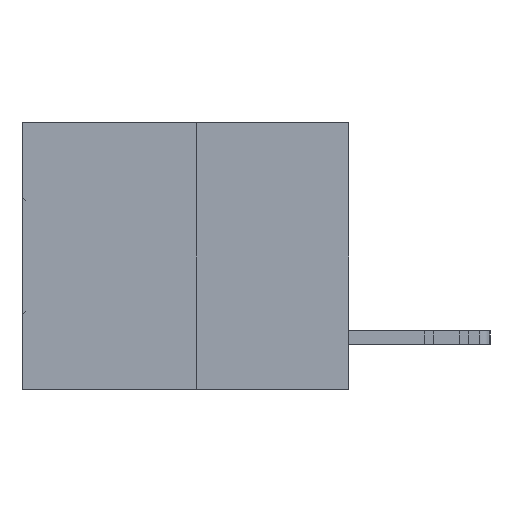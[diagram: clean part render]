
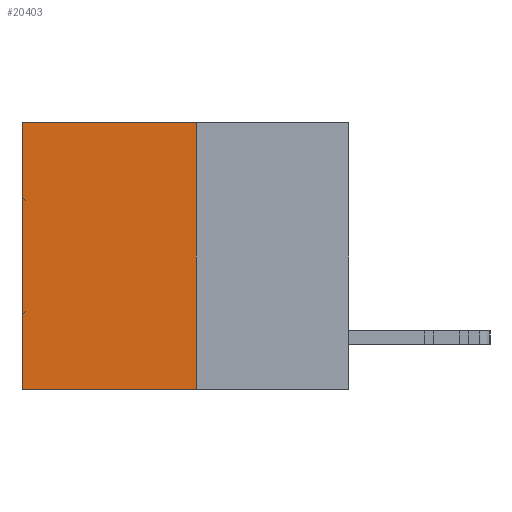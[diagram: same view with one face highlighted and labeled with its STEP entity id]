
A CAD part, left-side view. The second image highlights one B-rep face of the part: STEP entity #20403.
In plain terms, the highlighted planar face has unit normal (-1, 0, 0).
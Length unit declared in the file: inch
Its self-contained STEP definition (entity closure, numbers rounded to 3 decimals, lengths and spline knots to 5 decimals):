
#123 = LINE ( 'NONE', #18895, #16174 ) ;
#793 = CARTESIAN_POINT ( 'NONE',  ( 0.3165, 0.28, -0.49 ) ) ;
#831 = LINE ( 'NONE', #4594, #22726 ) ;
#1017 = LINE ( 'NONE', #18069, #3872 ) ;
#1722 = CARTESIAN_POINT ( 'NONE',  ( 0.3165, 0.6, -0.49 ) ) ;
#2252 = DIRECTION ( 'NONE',  ( 0., 0., -1. ) ) ;
#3872 = VECTOR ( 'NONE', #2252, 39.37008 ) ;
#4594 = CARTESIAN_POINT ( 'NONE',  ( 0.3165, 0.28, 0. ) ) ;
#9068 = VERTEX_POINT ( 'NONE', #22240 ) ;
#10817 = CARTESIAN_POINT ( 'NONE',  ( 0.3165, 0.28, -0.49 ) ) ;
#12361 = CARTESIAN_POINT ( 'NONE',  ( 0.3165, 0.28, 0. ) ) ;
#13529 = EDGE_LOOP ( 'NONE', ( #17844, #29411, #20712, #14182 ) ) ;
#13698 = VERTEX_POINT ( 'NONE', #14659 ) ;
#13804 = PLANE ( 'NONE',  #16335 ) ;
#14182 = ORIENTED_EDGE ( 'NONE', *, *, #19630, .T. ) ;
#14659 = CARTESIAN_POINT ( 'NONE',  ( 0.3165, 0.6, 0. ) ) ;
#15129 = EDGE_CURVE ( 'NONE', #34155, #26546, #1017, .T. ) ;
#15660 = VECTOR ( 'NONE', #21208, 39.37008 ) ;
#16174 = VECTOR ( 'NONE', #24242, 39.37008 ) ;
#16335 = AXIS2_PLACEMENT_3D ( 'NONE', #793, #19218, #21887 ) ;
#16602 = EDGE_CURVE ( 'NONE', #26546, #9068, #123, .T. ) ;
#17844 = ORIENTED_EDGE ( 'NONE', *, *, #31906, .T. ) ;
#18069 = CARTESIAN_POINT ( 'NONE',  ( 0.3165, 0.28, -0.49 ) ) ;
#18895 = CARTESIAN_POINT ( 'NONE',  ( 0.3165, 0.28, -0.49 ) ) ;
#19218 = DIRECTION ( 'NONE',  ( 1., 0., 0. ) ) ;
#19630 = EDGE_CURVE ( 'NONE', #34155, #13698, #831, .T. ) ;
#20403 = ADVANCED_FACE ( 'NONE', ( #25981 ), #13804, .F. ) ;
#20712 = ORIENTED_EDGE ( 'NONE', *, *, #15129, .F. ) ;
#21208 = DIRECTION ( 'NONE',  ( 0., 0., -1. ) ) ;
#21887 = DIRECTION ( 'NONE',  ( 0., 0., -1. ) ) ;
#22240 = CARTESIAN_POINT ( 'NONE',  ( 0.3165, 0.6, -0.49 ) ) ;
#22726 = VECTOR ( 'NONE', #28234, 39.37008 ) ;
#22733 = LINE ( 'NONE', #1722, #15660 ) ;
#24242 = DIRECTION ( 'NONE',  ( 0., 1., 0. ) ) ;
#25981 = FACE_OUTER_BOUND ( 'NONE', #13529, .T. ) ;
#26546 = VERTEX_POINT ( 'NONE', #10817 ) ;
#28234 = DIRECTION ( 'NONE',  ( 0., 1., 0. ) ) ;
#29411 = ORIENTED_EDGE ( 'NONE', *, *, #16602, .F. ) ;
#31906 = EDGE_CURVE ( 'NONE', #13698, #9068, #22733, .T. ) ;
#34155 = VERTEX_POINT ( 'NONE', #12361 ) ;
